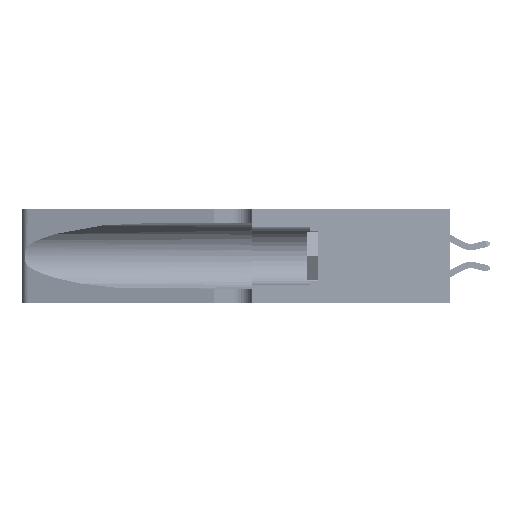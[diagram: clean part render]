
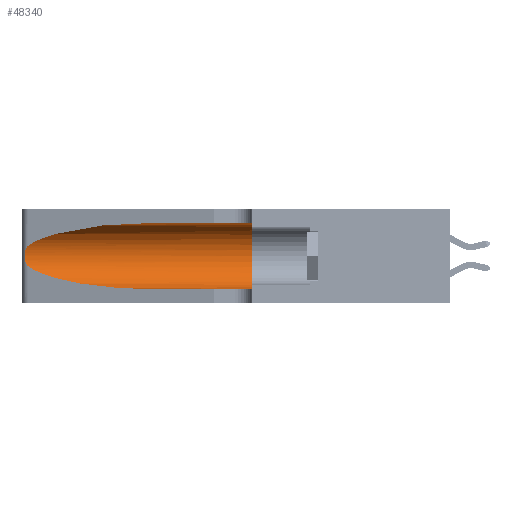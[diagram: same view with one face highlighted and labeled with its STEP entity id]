
A CAD part, left-side view. The second image highlights one B-rep face of the part: STEP entity #48340.
In plain terms, the highlighted cylindrical face has radius 3.308 mm (diameter 6.617 mm), a partial arc.
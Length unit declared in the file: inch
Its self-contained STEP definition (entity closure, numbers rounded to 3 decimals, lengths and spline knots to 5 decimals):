
#629 = CARTESIAN_POINT ( 'NONE',  ( 0.25487, 1.22718, 0.14631 ) ) ;
#813 = EDGE_CURVE ( 'NONE', #2905, #4787, #18145, .T. ) ;
#2605 = CARTESIAN_POINT ( 'NONE',  ( 0.1305, 1.61858, 0.185 ) ) ;
#2759 = CARTESIAN_POINT ( 'NONE',  ( 0.25856, 1.23593, 0.16098 ) ) ;
#2905 = VERTEX_POINT ( 'NONE', #15480 ) ;
#3898 = LINE ( 'NONE', #4444, #23270 ) ;
#4376 = VERTEX_POINT ( 'NONE', #5883 ) ;
#4444 = CARTESIAN_POINT ( 'NONE',  ( 0.1305, 1.61858, 0.31525 ) ) ;
#4787 = VERTEX_POINT ( 'NONE', #629 ) ;
#5421 = CARTESIAN_POINT ( 'NONE',  ( 0.1305, 0.35, 0.31525 ) ) ;
#5515 = ORIENTED_EDGE ( 'NONE', *, *, #11901, .T. ) ;
#5623 = CYLINDRICAL_SURFACE ( 'NONE', #26108, 0.13025 ) ;
#5759 = EDGE_LOOP ( 'NONE', ( #28446, #7746, #15780, #5515, #39313, #25557 ) ) ;
#5883 = CARTESIAN_POINT ( 'NONE',  ( 0.1305, 0.72297, 0.05475 ) ) ;
#6581 = EDGE_CURVE ( 'NONE', #4787, #4376, #44617, .T. ) ;
#6750 = CARTESIAN_POINT ( 'NONE',  ( 0.25639, 1.23186, 0.15144 ) ) ;
#7052 = EDGE_CURVE ( 'NONE', #12805, #49491, #30495, .T. ) ;
#7746 = ORIENTED_EDGE ( 'NONE', *, *, #813, .T. ) ;
#9714 = VECTOR ( 'NONE', #48227, 39.37008 ) ;
#10742 = CARTESIAN_POINT ( 'NONE',  ( 0.25487, 1.22718, 0.14631 ) ) ;
#11148 = CARTESIAN_POINT ( 'NONE',  ( 0.1305, 0.72297, 0.31525 ) ) ;
#11901 = EDGE_CURVE ( 'NONE', #4376, #49491, #40139, .T. ) ;
#12805 = VERTEX_POINT ( 'NONE', #5421 ) ;
#14481 = CARTESIAN_POINT ( 'NONE',  ( 0.25487, 1.22718, 0.22369 ) ) ;
#15480 = CARTESIAN_POINT ( 'NONE',  ( 0.25487, 1.22718, 0.22369 ) ) ;
#15780 = ORIENTED_EDGE ( 'NONE', *, *, #6581, .T. ) ;
#17347 = CARTESIAN_POINT ( 'NONE',  ( 0.1305, 0.35, 0.05475 ) ) ;
#17785 = EDGE_CURVE ( 'NONE', #38055, #2905, #39454, .T. ) ;
#18145 = B_SPLINE_CURVE_WITH_KNOTS ( 'NONE', 3,
 ( #14481, #21954, #37254, #41022, #18294, #44852, #22120, #48734, #25952, #2759, #29758, #6750, #33584, #10742 ),
 .UNSPECIFIED., .F., .F.,
 ( 4, 2, 2, 2, 2, 2, 4 ),
 ( 0., 0.00027, 0.00053, 0.00107, 0.0016, 0.00187, 0.00214 ),
 .UNSPECIFIED. ) ;
#18294 = CARTESIAN_POINT ( 'NONE',  ( 0.25854, 1.2359, 0.20912 ) ) ;
#20065 = DIRECTION ( 'NONE',  ( 0., 1., 0. ) ) ;
#20159 = CARTESIAN_POINT ( 'NONE',  ( 0.2373, 1.15595, 0.28018 ) ) ;
#21131 = CARTESIAN_POINT ( 'NONE',  ( 0.1305, 0.72297, 0.05475 ) ) ;
#21954 = CARTESIAN_POINT ( 'NONE',  ( 0.25555, 1.22994, 0.2215 ) ) ;
#22120 = CARTESIAN_POINT ( 'NONE',  ( 0.26075, 1.23896, 0.19203 ) ) ;
#23270 = VECTOR ( 'NONE', #23877, 39.37008 ) ;
#23877 = DIRECTION ( 'NONE',  ( 0., -1., 0. ) ) ;
#25557 = ORIENTED_EDGE ( 'NONE', *, *, #47324, .F. ) ;
#25952 = CARTESIAN_POINT ( 'NONE',  ( 0.26017, 1.23833, 0.17102 ) ) ;
#26108 = AXIS2_PLACEMENT_3D ( 'NONE', #2605, #48580, #29610 ) ;
#26138 = FACE_OUTER_BOUND ( 'NONE', #5759, .T. ) ;
#28446 = ORIENTED_EDGE ( 'NONE', *, *, #17785, .T. ) ;
#28625 = CARTESIAN_POINT ( 'NONE',  ( 0.25487, 1.22718, 0.14631 ) ) ;
#29610 = DIRECTION ( 'NONE',  ( 0., 0., -1. ) ) ;
#29758 = CARTESIAN_POINT ( 'NONE',  ( 0.25789, 1.23486, 0.15765 ) ) ;
#30495 = CIRCLE ( 'NONE', #49742, 0.13025 ) ;
#33584 = CARTESIAN_POINT ( 'NONE',  ( 0.25555, 1.22993, 0.14849 ) ) ;
#37254 = CARTESIAN_POINT ( 'NONE',  ( 0.25639, 1.23184, 0.21858 ) ) ;
#38055 = VERTEX_POINT ( 'NONE', #11148 ) ;
#39125 = CARTESIAN_POINT ( 'NONE',  ( 0.1305, 0.72297, 0.31525 ) ) ;
#39313 = ORIENTED_EDGE ( 'NONE', *, *, #7052, .F. ) ;
#39454 =( BOUNDED_CURVE ( )  B_SPLINE_CURVE ( 3, ( #39125, #42915, #20159, #46768 ),
 .UNSPECIFIED., .F., .F. ) 
 B_SPLINE_CURVE_WITH_KNOTS ( ( 4, 4 ),
 ( 1.5708, 2.84003 ),
 .UNSPECIFIED. ) 
 CURVE ( )  GEOMETRIC_REPRESENTATION_ITEM ( )  RATIONAL_B_SPLINE_CURVE ( ( 1., 0.87, 0.87, 1. ) ) 
 REPRESENTATION_ITEM ( '' )  );
#40139 = LINE ( 'NONE', #40525, #9714 ) ;
#40525 = CARTESIAN_POINT ( 'NONE',  ( 0.1305, 1.61858, 0.05475 ) ) ;
#41022 = CARTESIAN_POINT ( 'NONE',  ( 0.25787, 1.23484, 0.2124 ) ) ;
#42816 = CARTESIAN_POINT ( 'NONE',  ( 0.1305, 0.35, 0.185 ) ) ;
#42915 = CARTESIAN_POINT ( 'NONE',  ( 0.18966, 0.96281, 0.31525 ) ) ;
#43867 = CARTESIAN_POINT ( 'NONE',  ( 0.18966, 0.96281, 0.05475 ) ) ;
#44617 =( BOUNDED_CURVE ( )  B_SPLINE_CURVE ( 3, ( #28625, #47578, #43867, #21131 ),
 .UNSPECIFIED., .F., .F. ) 
 B_SPLINE_CURVE_WITH_KNOTS ( ( 4, 4 ),
 ( 3.44316, 4.71239 ),
 .UNSPECIFIED. ) 
 CURVE ( )  GEOMETRIC_REPRESENTATION_ITEM ( )  RATIONAL_B_SPLINE_CURVE ( ( 1., 0.87, 0.87, 1. ) ) 
 REPRESENTATION_ITEM ( '' )  );
#44852 = CARTESIAN_POINT ( 'NONE',  ( 0.26018, 1.23835, 0.19895 ) ) ;
#46669 = DIRECTION ( 'NONE',  ( 0., 0., 1. ) ) ;
#46768 = CARTESIAN_POINT ( 'NONE',  ( 0.25487, 1.22718, 0.22369 ) ) ;
#47324 = EDGE_CURVE ( 'NONE', #38055, #12805, #3898, .T. ) ;
#47578 = CARTESIAN_POINT ( 'NONE',  ( 0.2373, 1.15595, 0.08982 ) ) ;
#48227 = DIRECTION ( 'NONE',  ( 0., -1., 0. ) ) ;
#48340 = ADVANCED_FACE ( 'NONE', ( #26138 ), #5623, .F. ) ;
#48580 = DIRECTION ( 'NONE',  ( 0., -1., 0. ) ) ;
#48734 = CARTESIAN_POINT ( 'NONE',  ( 0.26075, 1.23896, 0.178 ) ) ;
#49491 = VERTEX_POINT ( 'NONE', #17347 ) ;
#49742 = AXIS2_PLACEMENT_3D ( 'NONE', #42816, #20065, #46669 ) ;
